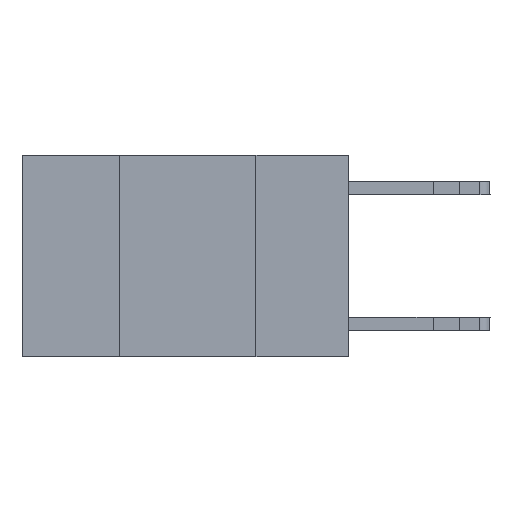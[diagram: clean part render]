
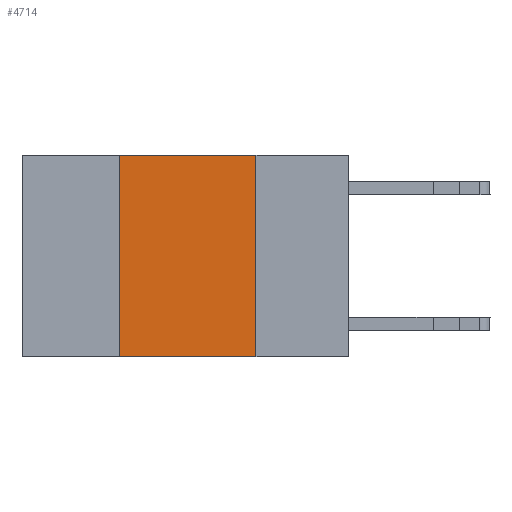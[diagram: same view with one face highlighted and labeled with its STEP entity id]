
A CAD part, left-side view. The second image highlights one B-rep face of the part: STEP entity #4714.
In plain terms, the highlighted planar face has unit normal (-1, 0, 0).
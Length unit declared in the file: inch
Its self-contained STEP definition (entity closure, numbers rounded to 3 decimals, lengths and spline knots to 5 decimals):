
#157 = VECTOR ( 'NONE', #18588, 39.37008 ) ;
#742 = CARTESIAN_POINT ( 'NONE',  ( 0., 0.6, 0. ) ) ;
#1979 = VECTOR ( 'NONE', #11290, 39.37008 ) ;
#2228 = LINE ( 'NONE', #4340, #157 ) ;
#2473 = CARTESIAN_POINT ( 'NONE',  ( 0., 0.42, 0. ) ) ;
#2596 = EDGE_CURVE ( 'NONE', #14634, #21594, #14949, .T. ) ;
#3316 = EDGE_CURVE ( 'NONE', #16213, #14634, #19651, .T. ) ;
#3780 = EDGE_CURVE ( 'NONE', #21594, #16788, #2228, .T. ) ;
#3840 = DIRECTION ( 'NONE',  ( 0., -1., 0. ) ) ;
#4318 = ORIENTED_EDGE ( 'NONE', *, *, #3316, .F. ) ;
#4340 = CARTESIAN_POINT ( 'NONE',  ( 0., 0.17, 0. ) ) ;
#4714 = ADVANCED_FACE ( 'NONE', ( #13051 ), #5843, .F. ) ;
#5344 = AXIS2_PLACEMENT_3D ( 'NONE', #742, #18660, #9751 ) ;
#5843 = PLANE ( 'NONE',  #5344 ) ;
#7748 = CARTESIAN_POINT ( 'NONE',  ( 0., 0.6, -0.37 ) ) ;
#8257 = ORIENTED_EDGE ( 'NONE', *, *, #16848, .T. ) ;
#9751 = DIRECTION ( 'NONE',  ( 0., 0., -1. ) ) ;
#10663 = VECTOR ( 'NONE', #3840, 39.37008 ) ;
#11138 = CARTESIAN_POINT ( 'NONE',  ( 0., 0.17, 0. ) ) ;
#11290 = DIRECTION ( 'NONE',  ( 0., -1., 0. ) ) ;
#13051 = FACE_OUTER_BOUND ( 'NONE', #22981, .T. ) ;
#14607 = ORIENTED_EDGE ( 'NONE', *, *, #2596, .F. ) ;
#14634 = VERTEX_POINT ( 'NONE', #2473 ) ;
#14949 = LINE ( 'NONE', #21983, #1979 ) ;
#15561 = CARTESIAN_POINT ( 'NONE',  ( 0., 0.42, -0.37 ) ) ;
#15865 = CARTESIAN_POINT ( 'NONE',  ( 0., 0.17, -0.37 ) ) ;
#16213 = VERTEX_POINT ( 'NONE', #15561 ) ;
#16788 = VERTEX_POINT ( 'NONE', #15865 ) ;
#16848 = EDGE_CURVE ( 'NONE', #16213, #16788, #18212, .T. ) ;
#18212 = LINE ( 'NONE', #7748, #10663 ) ;
#18588 = DIRECTION ( 'NONE',  ( 0., 0., -1. ) ) ;
#18660 = DIRECTION ( 'NONE',  ( 1., 0., 0. ) ) ;
#18780 = ORIENTED_EDGE ( 'NONE', *, *, #3780, .F. ) ;
#19651 = LINE ( 'NONE', #19767, #20083 ) ;
#19767 = CARTESIAN_POINT ( 'NONE',  ( 0., 0.42, 0. ) ) ;
#19891 = DIRECTION ( 'NONE',  ( 0., 0., 1. ) ) ;
#20083 = VECTOR ( 'NONE', #19891, 39.37008 ) ;
#21594 = VERTEX_POINT ( 'NONE', #11138 ) ;
#21983 = CARTESIAN_POINT ( 'NONE',  ( 0., 0.6, 0. ) ) ;
#22981 = EDGE_LOOP ( 'NONE', ( #18780, #14607, #4318, #8257 ) ) ;
